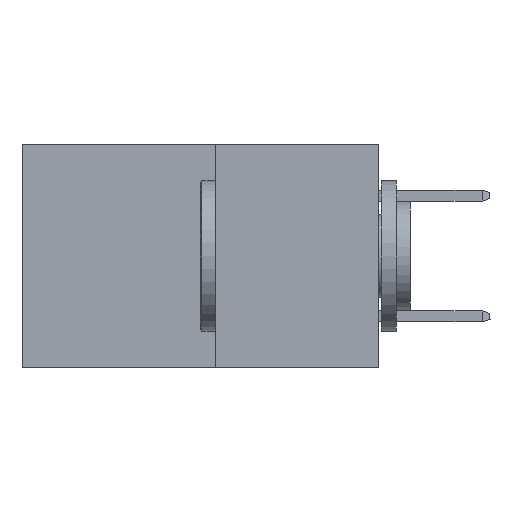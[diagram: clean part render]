
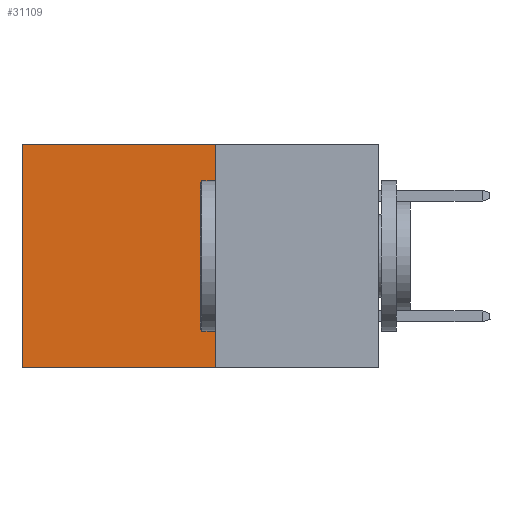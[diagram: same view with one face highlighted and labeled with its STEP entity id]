
A CAD part, left-side view. The second image highlights one B-rep face of the part: STEP entity #31109.
In plain terms, the highlighted planar face has unit normal (-1, 0, 0).
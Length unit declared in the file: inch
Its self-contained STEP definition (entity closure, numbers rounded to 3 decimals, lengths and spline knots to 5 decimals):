
#242 = FACE_OUTER_BOUND ( 'NONE', #11589, .T. ) ;
#1207 = VERTEX_POINT ( 'NONE', #16297 ) ;
#2043 = ORIENTED_EDGE ( 'NONE', *, *, #5518, .F. ) ;
#2654 = DIRECTION ( 'NONE',  ( 0., 0., -1. ) ) ;
#3689 = CARTESIAN_POINT ( 'NONE',  ( 0.277, 0.27, -0.37 ) ) ;
#4159 = DIRECTION ( 'NONE',  ( 0., 0., -1. ) ) ;
#4264 = CARTESIAN_POINT ( 'NONE',  ( 0.277, 0.27, -0.37 ) ) ;
#5031 = EDGE_CURVE ( 'NONE', #1207, #28478, #31229, .T. ) ;
#5518 = EDGE_CURVE ( 'NONE', #10596, #30722, #10687, .T. ) ;
#6113 = EDGE_CURVE ( 'NONE', #10596, #1207, #27115, .T. ) ;
#7669 = CARTESIAN_POINT ( 'NONE',  ( 0.277, 0.59, -0.37 ) ) ;
#7746 = CARTESIAN_POINT ( 'NONE',  ( 0.277, 0.27, -0.37 ) ) ;
#8348 = VECTOR ( 'NONE', #14296, 39.37008 ) ;
#10596 = VERTEX_POINT ( 'NONE', #25379 ) ;
#10687 = LINE ( 'NONE', #4264, #16647 ) ;
#11589 = EDGE_LOOP ( 'NONE', ( #27819, #21754, #2043, #19182 ) ) ;
#14296 = DIRECTION ( 'NONE',  ( 0., 1., 0. ) ) ;
#15389 = PLANE ( 'NONE',  #19991 ) ;
#15874 = LINE ( 'NONE', #22093, #8348 ) ;
#16297 = CARTESIAN_POINT ( 'NONE',  ( 0.277, 0.59, 0. ) ) ;
#16647 = VECTOR ( 'NONE', #4159, 39.37008 ) ;
#16788 = DIRECTION ( 'NONE',  ( 0., 0., -1. ) ) ;
#17984 = DIRECTION ( 'NONE',  ( 1., 0., 0. ) ) ;
#18328 = CARTESIAN_POINT ( 'NONE',  ( 0.277, 0.59, -0.37 ) ) ;
#18914 = DIRECTION ( 'NONE',  ( 0., 1., 0. ) ) ;
#19182 = ORIENTED_EDGE ( 'NONE', *, *, #6113, .T. ) ;
#19991 = AXIS2_PLACEMENT_3D ( 'NONE', #7746, #17984, #2654 ) ;
#20069 = CARTESIAN_POINT ( 'NONE',  ( 0.277, 0.27, 0. ) ) ;
#20290 = VECTOR ( 'NONE', #18914, 39.37008 ) ;
#21754 = ORIENTED_EDGE ( 'NONE', *, *, #30847, .F. ) ;
#22093 = CARTESIAN_POINT ( 'NONE',  ( 0.277, 0.27, -0.37 ) ) ;
#24391 = VECTOR ( 'NONE', #16788, 39.37008 ) ;
#25379 = CARTESIAN_POINT ( 'NONE',  ( 0.277, 0.27, 0. ) ) ;
#27115 = LINE ( 'NONE', #20069, #20290 ) ;
#27819 = ORIENTED_EDGE ( 'NONE', *, *, #5031, .T. ) ;
#28478 = VERTEX_POINT ( 'NONE', #7669 ) ;
#30722 = VERTEX_POINT ( 'NONE', #3689 ) ;
#30847 = EDGE_CURVE ( 'NONE', #30722, #28478, #15874, .T. ) ;
#31109 = ADVANCED_FACE ( 'NONE', ( #242 ), #15389, .F. ) ;
#31229 = LINE ( 'NONE', #18328, #24391 ) ;
